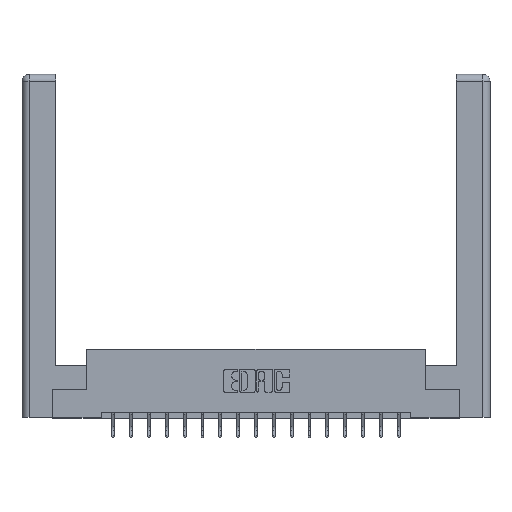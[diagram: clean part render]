
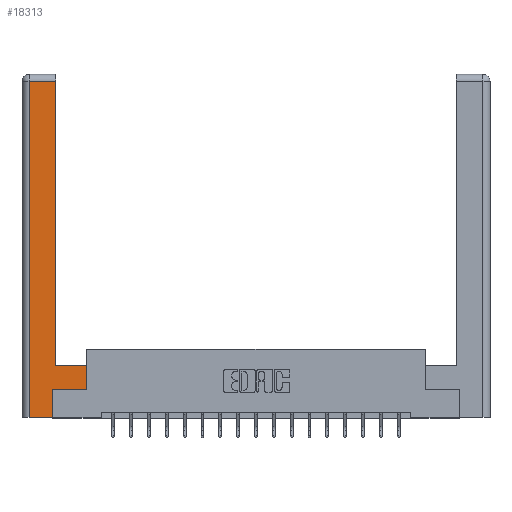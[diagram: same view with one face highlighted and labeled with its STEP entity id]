
A CAD part, top view. The second image highlights one B-rep face of the part: STEP entity #18313.
In plain terms, the highlighted planar face has unit normal (0, 0, 1).
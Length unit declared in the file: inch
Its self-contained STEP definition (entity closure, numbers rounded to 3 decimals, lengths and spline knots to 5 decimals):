
#17 = LINE ( 'NONE', #9608, #16095 ) ;
#45 = EDGE_CURVE ( 'NONE', #10215, #3895, #10147, .T. ) ;
#615 = DIRECTION ( 'NONE',  ( 0., 1., 0. ) ) ;
#797 = VERTEX_POINT ( 'NONE', #18260 ) ;
#1001 = EDGE_LOOP ( 'NONE', ( #14761, #16205, #7039, #13451, #14831, #14140, #18476, #5371 ) ) ;
#1007 = CARTESIAN_POINT ( 'NONE',  ( 0.295, 3., 0. ) ) ;
#1058 = VERTEX_POINT ( 'NONE', #4465 ) ;
#1299 = EDGE_CURVE ( 'NONE', #6450, #15648, #9398, .T. ) ;
#1401 = VECTOR ( 'NONE', #2514, 39.37008 ) ;
#1534 = DIRECTION ( 'NONE',  ( 1., 0., 0. ) ) ;
#1545 = EDGE_CURVE ( 'NONE', #1058, #10215, #17, .T. ) ;
#2319 = LINE ( 'NONE', #6278, #13295 ) ;
#2514 = DIRECTION ( 'NONE',  ( 0., 1., 0. ) ) ;
#3048 = CARTESIAN_POINT ( 'NONE',  ( 0.0615, 0., 0. ) ) ;
#3850 = EDGE_CURVE ( 'NONE', #16472, #797, #15093, .T. ) ;
#3895 = VERTEX_POINT ( 'NONE', #10139 ) ;
#4465 = CARTESIAN_POINT ( 'NONE',  ( 0.565, 0.245, 0. ) ) ;
#5371 = ORIENTED_EDGE ( 'NONE', *, *, #45, .T. ) ;
#5719 = VECTOR ( 'NONE', #1534, 39.37008 ) ;
#5911 = VECTOR ( 'NONE', #6521, 39.37008 ) ;
#6060 = LINE ( 'NONE', #1007, #1401 ) ;
#6278 = CARTESIAN_POINT ( 'NONE',  ( 0.265, 0.245, 0. ) ) ;
#6343 = DIRECTION ( 'NONE',  ( 0., 1., 0. ) ) ;
#6450 = VERTEX_POINT ( 'NONE', #16741 ) ;
#6461 = PLANE ( 'NONE',  #7529 ) ;
#6521 = DIRECTION ( 'NONE',  ( -1., 0., 0. ) ) ;
#6547 = CARTESIAN_POINT ( 'NONE',  ( 0.565, 0.45, 0. ) ) ;
#7039 = ORIENTED_EDGE ( 'NONE', *, *, #10767, .T. ) ;
#7529 = AXIS2_PLACEMENT_3D ( 'NONE', #12664, #16872, #7985 ) ;
#7838 = CARTESIAN_POINT ( 'NONE',  ( 0.0615, 0., 0. ) ) ;
#7985 = DIRECTION ( 'NONE',  ( -1., 0., 0. ) ) ;
#9294 = VECTOR ( 'NONE', #19119, 39.37008 ) ;
#9398 = LINE ( 'NONE', #16087, #12410 ) ;
#9529 = EDGE_CURVE ( 'NONE', #14839, #1058, #17125, .T. ) ;
#9608 = CARTESIAN_POINT ( 'NONE',  ( 0.565, 0.45, 0. ) ) ;
#10139 = CARTESIAN_POINT ( 'NONE',  ( 0.295, 0.45, 0. ) ) ;
#10147 = LINE ( 'NONE', #11167, #5911 ) ;
#10215 = VERTEX_POINT ( 'NONE', #6547 ) ;
#10513 = CARTESIAN_POINT ( 'NONE',  ( 0.565, 0.245, 0. ) ) ;
#10767 = EDGE_CURVE ( 'NONE', #15648, #16472, #15112, .T. ) ;
#11167 = CARTESIAN_POINT ( 'NONE',  ( 0.295, 0.45, 0. ) ) ;
#11519 = EDGE_CURVE ( 'NONE', #3895, #6450, #6060, .T. ) ;
#11694 = CARTESIAN_POINT ( 'NONE',  ( 0.265, 0., 0. ) ) ;
#12117 = VECTOR ( 'NONE', #13583, 39.37008 ) ;
#12410 = VECTOR ( 'NONE', #14673, 39.37008 ) ;
#12664 = CARTESIAN_POINT ( 'NONE',  ( 0., 0., 0. ) ) ;
#13295 = VECTOR ( 'NONE', #6343, 39.37008 ) ;
#13451 = ORIENTED_EDGE ( 'NONE', *, *, #3850, .T. ) ;
#13583 = DIRECTION ( 'NONE',  ( 0., -1., 0. ) ) ;
#14140 = ORIENTED_EDGE ( 'NONE', *, *, #9529, .T. ) ;
#14673 = DIRECTION ( 'NONE',  ( -1., 0., 0. ) ) ;
#14720 = FACE_OUTER_BOUND ( 'NONE', #1001, .T. ) ;
#14761 = ORIENTED_EDGE ( 'NONE', *, *, #11519, .T. ) ;
#14831 = ORIENTED_EDGE ( 'NONE', *, *, #18774, .T. ) ;
#14839 = VERTEX_POINT ( 'NONE', #17579 ) ;
#15093 = LINE ( 'NONE', #11694, #9294 ) ;
#15112 = LINE ( 'NONE', #7838, #12117 ) ;
#15648 = VERTEX_POINT ( 'NONE', #17107 ) ;
#16087 = CARTESIAN_POINT ( 'NONE',  ( 0.0615, 2.94, 0. ) ) ;
#16095 = VECTOR ( 'NONE', #615, 39.37008 ) ;
#16205 = ORIENTED_EDGE ( 'NONE', *, *, #1299, .T. ) ;
#16472 = VERTEX_POINT ( 'NONE', #3048 ) ;
#16741 = CARTESIAN_POINT ( 'NONE',  ( 0.295, 2.94, 0. ) ) ;
#16872 = DIRECTION ( 'NONE',  ( 0., 0., -1. ) ) ;
#17107 = CARTESIAN_POINT ( 'NONE',  ( 0.0615, 2.94, 0. ) ) ;
#17125 = LINE ( 'NONE', #10513, #5719 ) ;
#17579 = CARTESIAN_POINT ( 'NONE',  ( 0.265, 0.245, 0. ) ) ;
#18260 = CARTESIAN_POINT ( 'NONE',  ( 0.265, 0., 0. ) ) ;
#18313 = ADVANCED_FACE ( 'NONE', ( #14720 ), #6461, .F. ) ;
#18476 = ORIENTED_EDGE ( 'NONE', *, *, #1545, .T. ) ;
#18774 = EDGE_CURVE ( 'NONE', #797, #14839, #2319, .T. ) ;
#19119 = DIRECTION ( 'NONE',  ( 1., 0., 0. ) ) ;
